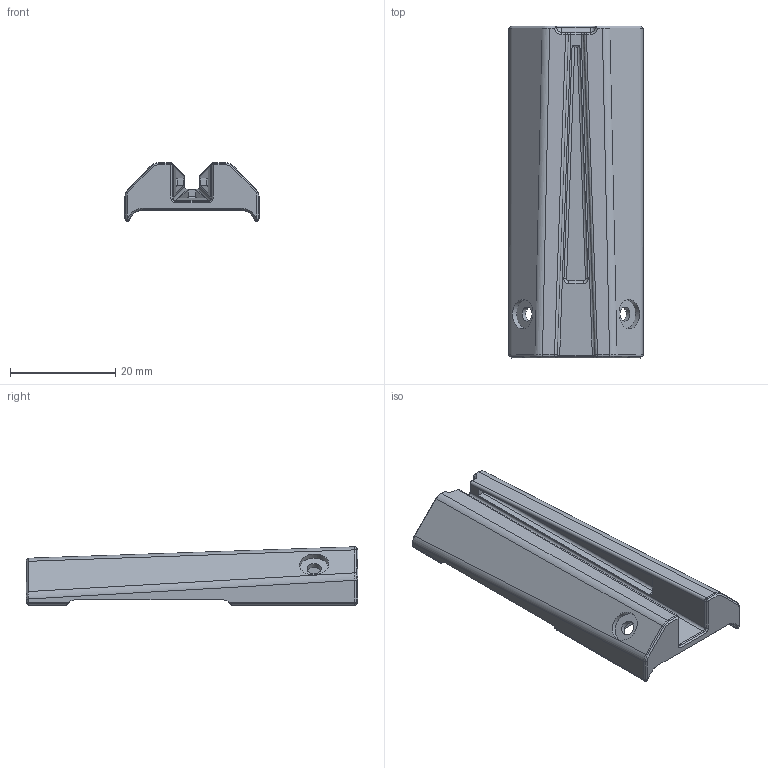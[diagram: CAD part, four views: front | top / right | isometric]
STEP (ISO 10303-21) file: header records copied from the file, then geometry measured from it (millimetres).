
FILE_DESCRIPTION(/* description */ (''),/* implementation_level */ '2;1');
FILE_NAME(/* name */ 'Sight Body.step',/* time_stamp */ '2021-06-23T20:35:16-04:00',/* author */ (''),/* organization */ (''),/* preprocessor_version */ 'ST-DEVELOPER v18.1',/* originating_system */ 'Autodesk Translation Framework v10.9.0.1377',/* authorisation */ '');
FILE_SCHEMA (('AUTOMOTIVE_DESIGN { 1 0 10303 214 3 1 1 }'));
Length unit declared in the file: millimetre
Products named in the file (1): Sight Body
Bounding box: 25.5 x 63.1 x 11.1 mm (x, y, z)
Volume: 5678.7 mm3; surface area: 7726 mm2
Topology: 1 solids, 3 shells, 384 faces, 952 edges, 569 vertices
Faces by surface type: bspline 132, plane 121, cylinder 87, cone 28, torus 10, sphere 6
Full cylindrical faces by diameter (mm): 2.7 x2, 5.6 x2
Entity records: 13554 total; most frequent: CARTESIAN_POINT 5178, ORIENTED_EDGE 1880, DIRECTION 1490, EDGE_CURVE 940, VERTEX_POINT 569, AXIS2_PLACEMENT_3D 531, LINE 428, VECTOR 428
